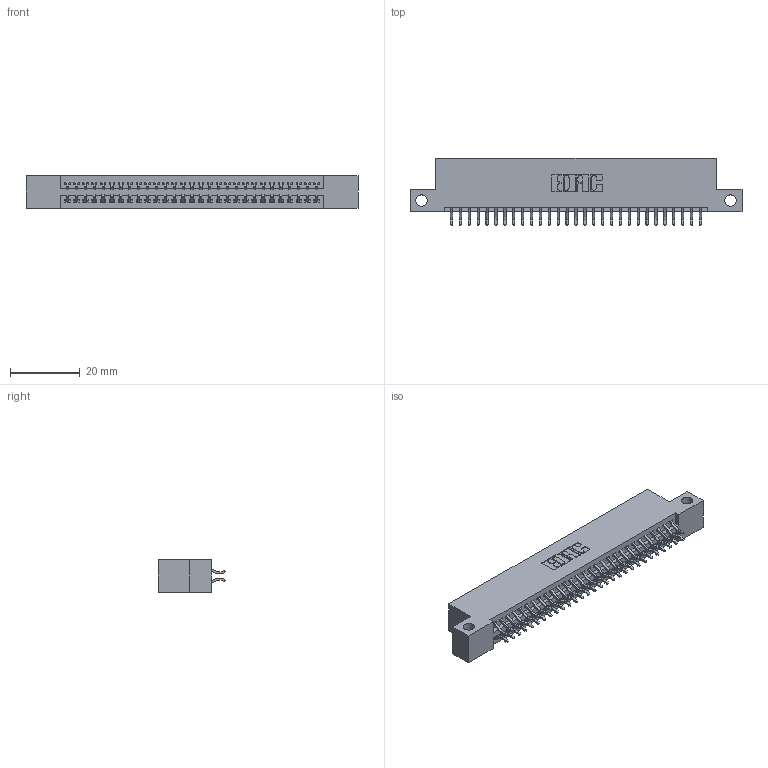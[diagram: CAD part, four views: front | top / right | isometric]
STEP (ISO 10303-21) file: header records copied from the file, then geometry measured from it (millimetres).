
FILE_DESCRIPTION (( 'STEP AP203' ), '1' );
FILE_NAME ('395-058-556-212.STEP', '2018-11-23T04:46:54', ( '' ), ( '' ), 'SwSTEP 2.0', 'SolidWorks 2016', '' );
FILE_SCHEMA (( 'CONFIG_CONTROL_DESIGN' ));
Length unit declared in the file: inch
Products named in the file (3): 395-058-556-212; 345 Part_Flush Mounting Lugs - Side Mount; 345-292-001_556 Tail
Assembly tree (59 placements, depth 2):
  395-058-556-212
    345 Part_Flush Mounting Lugs - Side Mount
    345-292-001_556 Tail  x58
Bounding box: 94.87 x 19.24 x 9.4 mm (x, y, z)
Volume: 9005.4 mm3; surface area: 12873.3 mm2
Topology: 59 solids, 59 shells, 3374 faces, 10027 edges, 6606 vertices
Faces by surface type: plane 2226, cylinder 1148
Entity records: 24727 total; most frequent: CARTESIAN_POINT 4172, ORIENTED_EDGE 4094, DIRECTION 3683, EDGE_CURVE 2047, LINE 1791, VECTOR 1791, VERTEX_POINT 1362, AXIS2_PLACEMENT_3D 946
